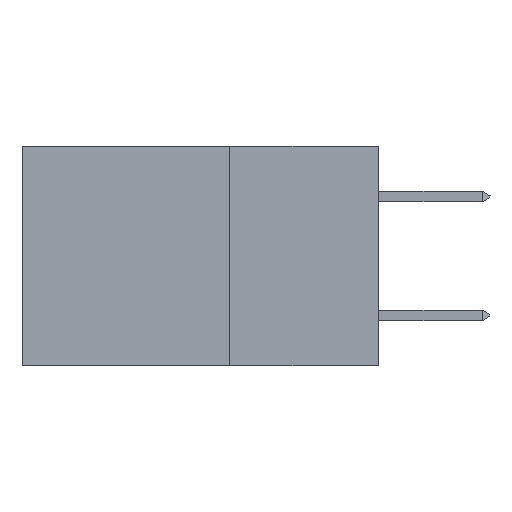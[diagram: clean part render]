
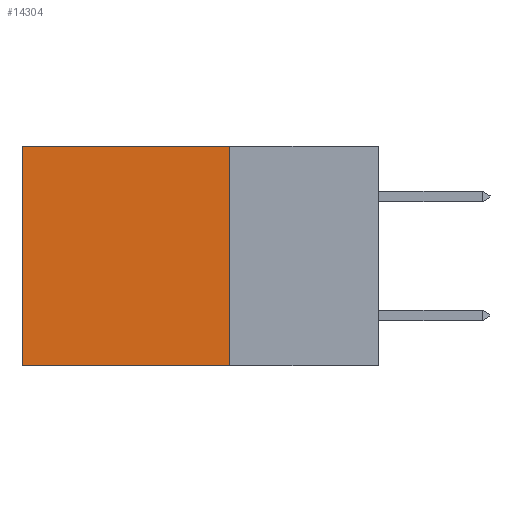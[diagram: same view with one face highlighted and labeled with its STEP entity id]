
A CAD part, left-side view. The second image highlights one B-rep face of the part: STEP entity #14304.
In plain terms, the highlighted planar face has unit normal (-1, 0, 0).
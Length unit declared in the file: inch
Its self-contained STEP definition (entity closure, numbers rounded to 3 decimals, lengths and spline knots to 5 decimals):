
#377 = DIRECTION ( 'NONE',  ( 0., 0., -1. ) ) ;
#390 = ORIENTED_EDGE ( 'NONE', *, *, #22182, .T. ) ;
#1561 = LINE ( 'NONE', #10627, #9796 ) ;
#1942 = ORIENTED_EDGE ( 'NONE', *, *, #11463, .F. ) ;
#2155 = VERTEX_POINT ( 'NONE', #14340 ) ;
#2488 = VERTEX_POINT ( 'NONE', #13590 ) ;
#3468 = VECTOR ( 'NONE', #17583, 39.37008 ) ;
#3505 = VECTOR ( 'NONE', #17201, 39.37008 ) ;
#3843 = DIRECTION ( 'NONE',  ( 1., 0., 0. ) ) ;
#4323 = VECTOR ( 'NONE', #20564, 39.37008 ) ;
#5850 = CARTESIAN_POINT ( 'NONE',  ( 0.2615, 0.25, 0. ) ) ;
#6505 = VERTEX_POINT ( 'NONE', #9915 ) ;
#9161 = EDGE_LOOP ( 'NONE', ( #390, #11383, #1942, #15325 ) ) ;
#9589 = LINE ( 'NONE', #18755, #4323 ) ;
#9596 = EDGE_CURVE ( 'NONE', #2488, #6505, #11860, .T. ) ;
#9796 = VECTOR ( 'NONE', #17759, 39.37008 ) ;
#9915 = CARTESIAN_POINT ( 'NONE',  ( 0.2615, 0.6, -0.37 ) ) ;
#10627 = CARTESIAN_POINT ( 'NONE',  ( 0.2615, 0.6, -0.37 ) ) ;
#10863 = VERTEX_POINT ( 'NONE', #5850 ) ;
#11335 = FACE_OUTER_BOUND ( 'NONE', #9161, .T. ) ;
#11383 = ORIENTED_EDGE ( 'NONE', *, *, #9596, .F. ) ;
#11463 = EDGE_CURVE ( 'NONE', #10863, #2488, #13745, .T. ) ;
#11860 = LINE ( 'NONE', #17226, #3468 ) ;
#13009 = PLANE ( 'NONE',  #20727 ) ;
#13590 = CARTESIAN_POINT ( 'NONE',  ( 0.2615, 0.25, -0.37 ) ) ;
#13745 = LINE ( 'NONE', #17554, #3505 ) ;
#14304 = ADVANCED_FACE ( 'NONE', ( #11335 ), #13009, .F. ) ;
#14340 = CARTESIAN_POINT ( 'NONE',  ( 0.2615, 0.6, 0. ) ) ;
#15197 = EDGE_CURVE ( 'NONE', #10863, #2155, #9589, .T. ) ;
#15325 = ORIENTED_EDGE ( 'NONE', *, *, #15197, .T. ) ;
#16819 = CARTESIAN_POINT ( 'NONE',  ( 0.2615, 0.25, -0.37 ) ) ;
#17201 = DIRECTION ( 'NONE',  ( 0., 0., -1. ) ) ;
#17226 = CARTESIAN_POINT ( 'NONE',  ( 0.2615, 0.25, -0.37 ) ) ;
#17554 = CARTESIAN_POINT ( 'NONE',  ( 0.2615, 0.25, -0.37 ) ) ;
#17583 = DIRECTION ( 'NONE',  ( 0., 1., 0. ) ) ;
#17759 = DIRECTION ( 'NONE',  ( 0., 0., -1. ) ) ;
#18755 = CARTESIAN_POINT ( 'NONE',  ( 0.2615, 0.25, 0. ) ) ;
#20564 = DIRECTION ( 'NONE',  ( 0., 1., 0. ) ) ;
#20727 = AXIS2_PLACEMENT_3D ( 'NONE', #16819, #3843, #377 ) ;
#22182 = EDGE_CURVE ( 'NONE', #2155, #6505, #1561, .T. ) ;
